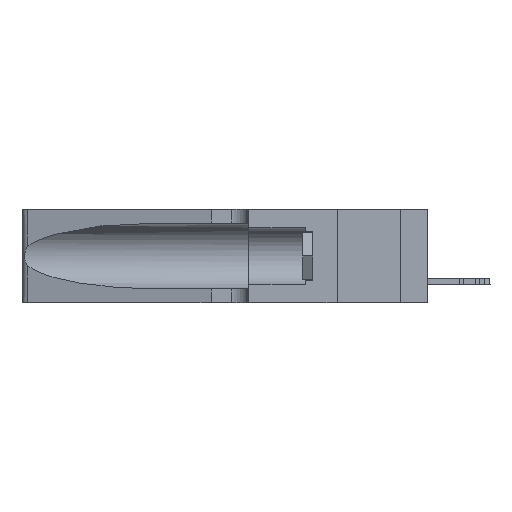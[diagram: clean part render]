
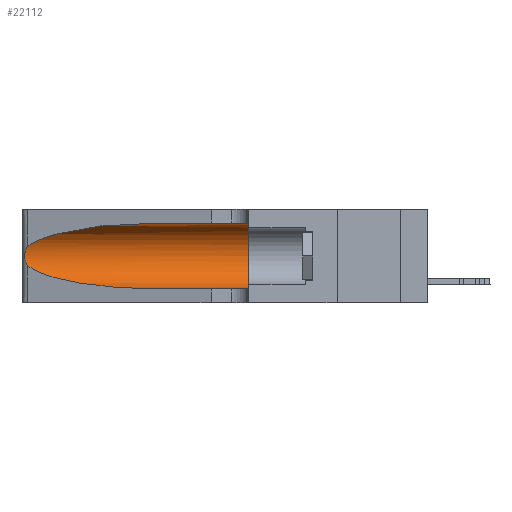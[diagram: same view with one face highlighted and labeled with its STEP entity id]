
A CAD part, left-side view. The second image highlights one B-rep face of the part: STEP entity #22112.
In plain terms, the highlighted cylindrical face has radius 3.308 mm (diameter 6.617 mm), a partial arc.
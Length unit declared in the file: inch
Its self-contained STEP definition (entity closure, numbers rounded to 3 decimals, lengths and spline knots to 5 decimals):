
#1565 = CARTESIAN_POINT ( 'NONE',  ( 0.25487, 1.22718, 0.22369 ) ) ;
#2084 = CARTESIAN_POINT ( 'NONE',  ( 0.1305, 0.72297, 0.05475 ) ) ;
#2472 = EDGE_CURVE ( 'NONE', #18353, #21748, #12709, .T. ) ;
#3165 = CARTESIAN_POINT ( 'NONE',  ( 0.25639, 1.23184, 0.21858 ) ) ;
#3225 = CYLINDRICAL_SURFACE ( 'NONE', #4920, 0.13025 ) ;
#3804 = DIRECTION ( 'NONE',  ( 0., 1., 0. ) ) ;
#4920 = AXIS2_PLACEMENT_3D ( 'NONE', #31612, #5664, #20504 ) ;
#5022 = ORIENTED_EDGE ( 'NONE', *, *, #9134, .T. ) ;
#5099 = CARTESIAN_POINT ( 'NONE',  ( 0.26017, 1.23833, 0.17102 ) ) ;
#5182 = VERTEX_POINT ( 'NONE', #42002 ) ;
#5472 = CARTESIAN_POINT ( 'NONE',  ( 0.2373, 1.15595, 0.28018 ) ) ;
#5664 = DIRECTION ( 'NONE',  ( 0., -1., 0. ) ) ;
#6456 = CARTESIAN_POINT ( 'NONE',  ( 0.2373, 1.15595, 0.08982 ) ) ;
#7447 = DIRECTION ( 'NONE',  ( 0., -1., 0. ) ) ;
#8779 = CARTESIAN_POINT ( 'NONE',  ( 0.25639, 1.23186, 0.15144 ) ) ;
#9134 = EDGE_CURVE ( 'NONE', #38503, #21748, #44956, .T. ) ;
#9455 = DIRECTION ( 'NONE',  ( 0., -1., 0. ) ) ;
#10077 = EDGE_CURVE ( 'NONE', #20216, #18353, #37953, .T. ) ;
#10370 = CARTESIAN_POINT ( 'NONE',  ( 0.1305, 0.72297, 0.31525 ) ) ;
#10589 = CARTESIAN_POINT ( 'NONE',  ( 0.25787, 1.23484, 0.2124 ) ) ;
#11648 = CARTESIAN_POINT ( 'NONE',  ( 0.25487, 1.22718, 0.22369 ) ) ;
#12036 = ORIENTED_EDGE ( 'NONE', *, *, #2472, .F. ) ;
#12083 = CARTESIAN_POINT ( 'NONE',  ( 0.1305, 0.72297, 0.05475 ) ) ;
#12208 = AXIS2_PLACEMENT_3D ( 'NONE', #33185, #3804, #18331 ) ;
#12625 = ORIENTED_EDGE ( 'NONE', *, *, #14315, .T. ) ;
#12709 = CIRCLE ( 'NONE', #12208, 0.13025 ) ;
#12717 = CARTESIAN_POINT ( 'NONE',  ( 0.18966, 0.96281, 0.31525 ) ) ;
#14315 = EDGE_CURVE ( 'NONE', #28438, #5182, #37566, .T. ) ;
#15749 =( BOUNDED_CURVE ( )  B_SPLINE_CURVE ( 3, ( #42801, #12717, #5472, #1565 ),
 .UNSPECIFIED., .F., .F. ) 
 B_SPLINE_CURVE_WITH_KNOTS ( ( 4, 4 ),
 ( 1.5708, 2.84003 ),
 .UNSPECIFIED. ) 
 CURVE ( )  GEOMETRIC_REPRESENTATION_ITEM ( )  RATIONAL_B_SPLINE_CURVE ( ( 1., 0.87, 0.87, 1. ) ) 
 REPRESENTATION_ITEM ( '' )  );
#16557 = CARTESIAN_POINT ( 'NONE',  ( 0.25789, 1.23486, 0.15765 ) ) ;
#18331 = DIRECTION ( 'NONE',  ( 0., 0., 1. ) ) ;
#18353 = VERTEX_POINT ( 'NONE', #26667 ) ;
#19919 = CARTESIAN_POINT ( 'NONE',  ( 0.25555, 1.22993, 0.14849 ) ) ;
#20216 = VERTEX_POINT ( 'NONE', #10370 ) ;
#20260 = CARTESIAN_POINT ( 'NONE',  ( 0.25487, 1.22718, 0.14631 ) ) ;
#20504 = DIRECTION ( 'NONE',  ( 0., 0., -1. ) ) ;
#21025 = CARTESIAN_POINT ( 'NONE',  ( 0.1305, 1.61858, 0.05475 ) ) ;
#21677 = VECTOR ( 'NONE', #7447, 39.37008 ) ;
#21748 = VERTEX_POINT ( 'NONE', #22432 ) ;
#22082 = CARTESIAN_POINT ( 'NONE',  ( 0.26018, 1.23835, 0.19895 ) ) ;
#22112 = ADVANCED_FACE ( 'NONE', ( #39877 ), #3225, .F. ) ;
#22432 = CARTESIAN_POINT ( 'NONE',  ( 0.1305, 0.35, 0.05475 ) ) ;
#23275 = EDGE_CURVE ( 'NONE', #5182, #38503, #33977, .T. ) ;
#26667 = CARTESIAN_POINT ( 'NONE',  ( 0.1305, 0.35, 0.31525 ) ) ;
#27144 = EDGE_CURVE ( 'NONE', #20216, #28438, #15749, .T. ) ;
#28438 = VERTEX_POINT ( 'NONE', #11648 ) ;
#28665 = ORIENTED_EDGE ( 'NONE', *, *, #23275, .T. ) ;
#29447 = ORIENTED_EDGE ( 'NONE', *, *, #10077, .F. ) ;
#31043 = CARTESIAN_POINT ( 'NONE',  ( 0.25856, 1.23593, 0.16098 ) ) ;
#31612 = CARTESIAN_POINT ( 'NONE',  ( 0.1305, 1.61858, 0.185 ) ) ;
#33185 = CARTESIAN_POINT ( 'NONE',  ( 0.1305, 0.35, 0.185 ) ) ;
#33977 =( BOUNDED_CURVE ( )  B_SPLINE_CURVE ( 3, ( #39625, #6456, #46671, #2084 ),
 .UNSPECIFIED., .F., .F. ) 
 B_SPLINE_CURVE_WITH_KNOTS ( ( 4, 4 ),
 ( 3.44316, 4.71239 ),
 .UNSPECIFIED. ) 
 CURVE ( )  GEOMETRIC_REPRESENTATION_ITEM ( )  RATIONAL_B_SPLINE_CURVE ( ( 1., 0.87, 0.87, 1. ) ) 
 REPRESENTATION_ITEM ( '' )  );
#36785 = VECTOR ( 'NONE', #9455, 39.37008 ) ;
#37566 = B_SPLINE_CURVE_WITH_KNOTS ( 'NONE', 3,
 ( #43909, #47605, #3165, #10589, #47923, #22082, #42119, #38903, #5099, #31043, #16557, #8779, #19919, #20260 ),
 .UNSPECIFIED., .F., .F.,
 ( 4, 2, 2, 2, 2, 2, 4 ),
 ( 0., 0.00027, 0.00053, 0.00107, 0.0016, 0.00187, 0.00214 ),
 .UNSPECIFIED. ) ;
#37953 = LINE ( 'NONE', #39110, #36785 ) ;
#38503 = VERTEX_POINT ( 'NONE', #12083 ) ;
#38903 = CARTESIAN_POINT ( 'NONE',  ( 0.26075, 1.23896, 0.178 ) ) ;
#39110 = CARTESIAN_POINT ( 'NONE',  ( 0.1305, 1.61858, 0.31525 ) ) ;
#39625 = CARTESIAN_POINT ( 'NONE',  ( 0.25487, 1.22718, 0.14631 ) ) ;
#39877 = FACE_OUTER_BOUND ( 'NONE', #40054, .T. ) ;
#40054 = EDGE_LOOP ( 'NONE', ( #43941, #12625, #28665, #5022, #12036, #29447 ) ) ;
#42002 = CARTESIAN_POINT ( 'NONE',  ( 0.25487, 1.22718, 0.14631 ) ) ;
#42119 = CARTESIAN_POINT ( 'NONE',  ( 0.26075, 1.23896, 0.19203 ) ) ;
#42801 = CARTESIAN_POINT ( 'NONE',  ( 0.1305, 0.72297, 0.31525 ) ) ;
#43909 = CARTESIAN_POINT ( 'NONE',  ( 0.25487, 1.22718, 0.22369 ) ) ;
#43941 = ORIENTED_EDGE ( 'NONE', *, *, #27144, .T. ) ;
#44956 = LINE ( 'NONE', #21025, #21677 ) ;
#46671 = CARTESIAN_POINT ( 'NONE',  ( 0.18966, 0.96281, 0.05475 ) ) ;
#47605 = CARTESIAN_POINT ( 'NONE',  ( 0.25555, 1.22994, 0.2215 ) ) ;
#47923 = CARTESIAN_POINT ( 'NONE',  ( 0.25854, 1.2359, 0.20912 ) ) ;
